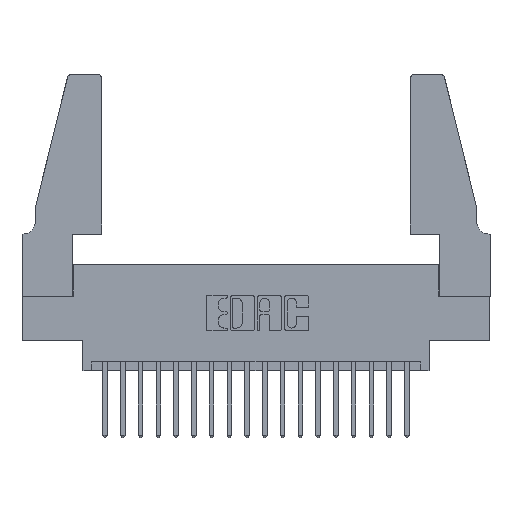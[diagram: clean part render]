
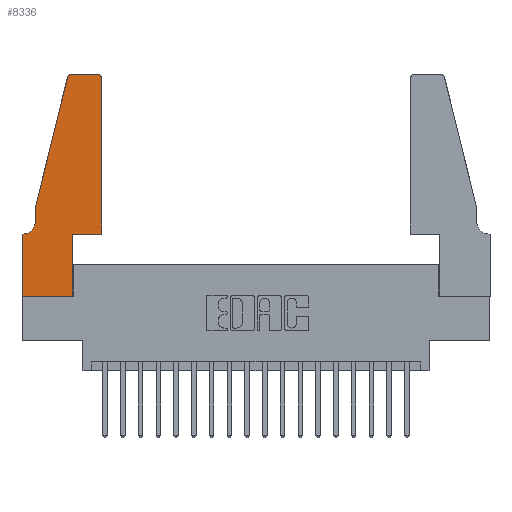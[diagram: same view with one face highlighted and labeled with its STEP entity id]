
A CAD part, top view. The second image highlights one B-rep face of the part: STEP entity #8336.
In plain terms, the highlighted planar face has unit normal (0, 0, 1).
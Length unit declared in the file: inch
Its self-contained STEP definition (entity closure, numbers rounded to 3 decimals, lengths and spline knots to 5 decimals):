
#337 = LINE ( 'NONE', #15535, #16127 ) ;
#463 = VECTOR ( 'NONE', #4334, 39.37008 ) ;
#514 = CARTESIAN_POINT ( 'NONE',  ( 0.25487, 1.22718, 0.37 ) ) ;
#915 = DIRECTION ( 'NONE',  ( -1., 0., 0. ) ) ;
#1209 = ORIENTED_EDGE ( 'NONE', *, *, #4247, .T. ) ;
#1420 = DIRECTION ( 'NONE',  ( 0., 0., 1. ) ) ;
#1549 = CARTESIAN_POINT ( 'NONE',  ( 0.4505, 1.22, 0.37 ) ) ;
#2165 = DIRECTION ( 'NONE',  ( 0., -1., 0. ) ) ;
#2747 = CARTESIAN_POINT ( 'NONE',  ( 0.4505, 0.35, 0.37 ) ) ;
#2772 = PLANE ( 'NONE',  #4694 ) ;
#2999 = VECTOR ( 'NONE', #10732, 39.37008 ) ;
#3678 = VERTEX_POINT ( 'NONE', #15746 ) ;
#3864 = ORIENTED_EDGE ( 'NONE', *, *, #11877, .T. ) ;
#3999 = CARTESIAN_POINT ( 'NONE',  ( 0.2865, 0.35, 0.37 ) ) ;
#4247 = EDGE_CURVE ( 'NONE', #12417, #12911, #337, .T. ) ;
#4329 = LINE ( 'NONE', #5384, #15985 ) ;
#4334 = DIRECTION ( 'NONE',  ( 0., 1., 0. ) ) ;
#4363 = DIRECTION ( 'NONE',  ( 1., 0., 0. ) ) ;
#4483 = LINE ( 'NONE', #12056, #16117 ) ;
#4631 = AXIS2_PLACEMENT_3D ( 'NONE', #4832, #15470, #6441 ) ;
#4694 = AXIS2_PLACEMENT_3D ( 'NONE', #12064, #13558, #4363 ) ;
#4763 = DIRECTION ( 'NONE',  ( 0., 1., 0. ) ) ;
#4832 = CARTESIAN_POINT ( 'NONE',  ( 0.0055, 0.42, 0.37 ) ) ;
#4904 = VERTEX_POINT ( 'NONE', #514 ) ;
#5132 = ORIENTED_EDGE ( 'NONE', *, *, #7077, .T. ) ;
#5308 = CARTESIAN_POINT ( 'NONE',  ( 0.0755, 0.5, 0.37 ) ) ;
#5374 = ORIENTED_EDGE ( 'NONE', *, *, #11941, .T. ) ;
#5384 = CARTESIAN_POINT ( 'NONE',  ( 0.2605, 1.25, 0.37 ) ) ;
#5408 = ORIENTED_EDGE ( 'NONE', *, *, #17999, .T. ) ;
#5756 = VERTEX_POINT ( 'NONE', #16126 ) ;
#6024 = LINE ( 'NONE', #13945, #18038 ) ;
#6065 = EDGE_CURVE ( 'NONE', #19485, #15135, #11200, .T. ) ;
#6086 = ORIENTED_EDGE ( 'NONE', *, *, #17893, .T. ) ;
#6441 = DIRECTION ( 'NONE',  ( -1., 0., 0. ) ) ;
#6619 = ORIENTED_EDGE ( 'NONE', *, *, #6923, .T. ) ;
#6834 = CARTESIAN_POINT ( 'NONE',  ( 0.2865, 0., 0.37 ) ) ;
#6923 = EDGE_CURVE ( 'NONE', #5756, #16963, #15573, .T. ) ;
#7077 = EDGE_CURVE ( 'NONE', #12911, #19485, #8776, .T. ) ;
#7256 = ORIENTED_EDGE ( 'NONE', *, *, #9666, .T. ) ;
#7664 = CARTESIAN_POINT ( 'NONE',  ( 0.0755, 0.5, 0.37 ) ) ;
#7808 = DIRECTION ( 'NONE',  ( 0., 0., 1. ) ) ;
#8057 = CARTESIAN_POINT ( 'NONE',  ( 0., 0., 0.37 ) ) ;
#8336 = ADVANCED_FACE ( 'NONE', ( #18062 ), #2772, .T. ) ;
#8466 = CIRCLE ( 'NONE', #18197, 0.03 ) ;
#8590 = EDGE_CURVE ( 'NONE', #16963, #14985, #13438, .T. ) ;
#8776 = LINE ( 'NONE', #2747, #463 ) ;
#9267 = EDGE_LOOP ( 'NONE', ( #19096, #6086, #5374, #7256, #18482, #6619, #10170, #3864, #5408, #1209, #5132, #13164 ) ) ;
#9585 = DIRECTION ( 'NONE',  ( 0., -1., 0. ) ) ;
#9666 = EDGE_CURVE ( 'NONE', #12210, #3678, #14341, .T. ) ;
#9891 = CARTESIAN_POINT ( 'NONE',  ( 0., 0.35, 0.37 ) ) ;
#10170 = ORIENTED_EDGE ( 'NONE', *, *, #8590, .T. ) ;
#10526 = AXIS2_PLACEMENT_3D ( 'NONE', #16781, #7808, #18260 ) ;
#10732 = DIRECTION ( 'NONE',  ( -0.239, -0.971, 0. ) ) ;
#10736 = CARTESIAN_POINT ( 'NONE',  ( 0.284, 1.22, 0.37 ) ) ;
#11161 = VECTOR ( 'NONE', #915, 39.37008 ) ;
#11200 = CIRCLE ( 'NONE', #10526, 0.03 ) ;
#11508 = CARTESIAN_POINT ( 'NONE',  ( 0., 0., 0.37 ) ) ;
#11877 = EDGE_CURVE ( 'NONE', #14985, #16296, #4483, .T. ) ;
#11941 = EDGE_CURVE ( 'NONE', #4904, #12210, #19112, .T. ) ;
#12056 = CARTESIAN_POINT ( 'NONE',  ( 0., 0., 0.37 ) ) ;
#12064 = CARTESIAN_POINT ( 'NONE',  ( 0., 0.35, 0.37 ) ) ;
#12210 = VERTEX_POINT ( 'NONE', #17221 ) ;
#12260 = DIRECTION ( 'NONE',  ( 1., 0., 0. ) ) ;
#12417 = VERTEX_POINT ( 'NONE', #3999 ) ;
#12647 = DIRECTION ( 'NONE',  ( 1., 0., 0. ) ) ;
#12911 = VERTEX_POINT ( 'NONE', #13860 ) ;
#13164 = ORIENTED_EDGE ( 'NONE', *, *, #6065, .T. ) ;
#13438 = LINE ( 'NONE', #8057, #13905 ) ;
#13558 = DIRECTION ( 'NONE',  ( 0., 0., 1. ) ) ;
#13860 = CARTESIAN_POINT ( 'NONE',  ( 0.4505, 0.35, 0.37 ) ) ;
#13890 = VECTOR ( 'NONE', #2165, 39.37008 ) ;
#13905 = VECTOR ( 'NONE', #9585, 39.37008 ) ;
#13945 = CARTESIAN_POINT ( 'NONE',  ( 0.2865, 0.35, 0.37 ) ) ;
#14119 = CIRCLE ( 'NONE', #4631, 0.07 ) ;
#14341 = LINE ( 'NONE', #5308, #13890 ) ;
#14985 = VERTEX_POINT ( 'NONE', #11508 ) ;
#15135 = VERTEX_POINT ( 'NONE', #16214 ) ;
#15470 = DIRECTION ( 'NONE',  ( 0., 0., -1. ) ) ;
#15535 = CARTESIAN_POINT ( 'NONE',  ( 0.4505, 0.35, 0.37 ) ) ;
#15573 = LINE ( 'NONE', #17664, #11161 ) ;
#15613 = VERTEX_POINT ( 'NONE', #18462 ) ;
#15746 = CARTESIAN_POINT ( 'NONE',  ( 0.0755, 0.42, 0.37 ) ) ;
#15864 = EDGE_CURVE ( 'NONE', #15135, #15613, #4329, .T. ) ;
#15985 = VECTOR ( 'NONE', #16000, 39.37008 ) ;
#16000 = DIRECTION ( 'NONE',  ( -1., 0., 0. ) ) ;
#16117 = VECTOR ( 'NONE', #17942, 39.37008 ) ;
#16126 = CARTESIAN_POINT ( 'NONE',  ( 0.0055, 0.35, 0.37 ) ) ;
#16127 = VECTOR ( 'NONE', #12647, 39.37008 ) ;
#16214 = CARTESIAN_POINT ( 'NONE',  ( 0.4205, 1.25, 0.37 ) ) ;
#16296 = VERTEX_POINT ( 'NONE', #6834 ) ;
#16781 = CARTESIAN_POINT ( 'NONE',  ( 0.4205, 1.22, 0.37 ) ) ;
#16963 = VERTEX_POINT ( 'NONE', #9891 ) ;
#17221 = CARTESIAN_POINT ( 'NONE',  ( 0.0755, 0.5, 0.37 ) ) ;
#17664 = CARTESIAN_POINT ( 'NONE',  ( 0.0755, 0.35, 0.37 ) ) ;
#17893 = EDGE_CURVE ( 'NONE', #15613, #4904, #8466, .T. ) ;
#17942 = DIRECTION ( 'NONE',  ( 1., 0., 0. ) ) ;
#17999 = EDGE_CURVE ( 'NONE', #16296, #12417, #6024, .T. ) ;
#18028 = EDGE_CURVE ( 'NONE', #3678, #5756, #14119, .T. ) ;
#18038 = VECTOR ( 'NONE', #4763, 39.37008 ) ;
#18062 = FACE_OUTER_BOUND ( 'NONE', #9267, .T. ) ;
#18197 = AXIS2_PLACEMENT_3D ( 'NONE', #10736, #1420, #12260 ) ;
#18260 = DIRECTION ( 'NONE',  ( 1., 0., 0. ) ) ;
#18462 = CARTESIAN_POINT ( 'NONE',  ( 0.284, 1.25, 0.37 ) ) ;
#18482 = ORIENTED_EDGE ( 'NONE', *, *, #18028, .T. ) ;
#19096 = ORIENTED_EDGE ( 'NONE', *, *, #15864, .T. ) ;
#19112 = LINE ( 'NONE', #7664, #2999 ) ;
#19485 = VERTEX_POINT ( 'NONE', #1549 ) ;
